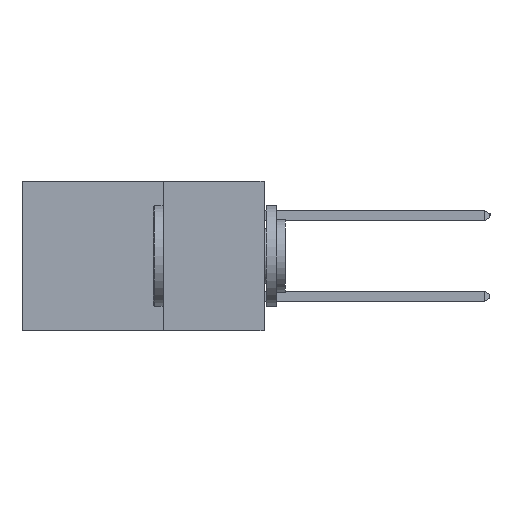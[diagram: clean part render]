
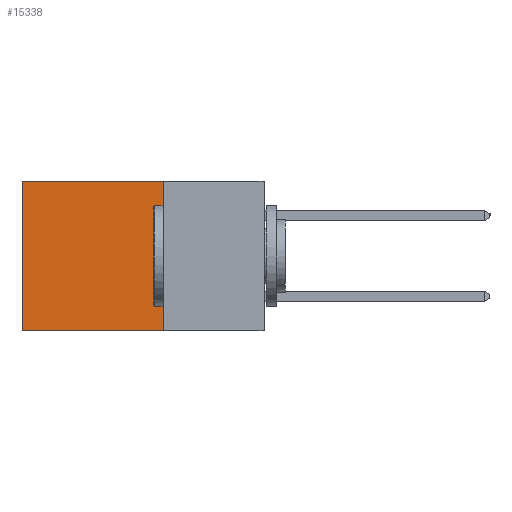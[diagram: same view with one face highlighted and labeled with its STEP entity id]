
A CAD part, left-side view. The second image highlights one B-rep face of the part: STEP entity #15338.
In plain terms, the highlighted planar face has unit normal (-1, 0, 0).
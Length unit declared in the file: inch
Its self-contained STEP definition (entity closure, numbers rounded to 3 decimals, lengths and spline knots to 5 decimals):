
#253 = LINE ( 'NONE', #8938, #17977 ) ;
#341 = VERTEX_POINT ( 'NONE', #9556 ) ;
#1748 = DIRECTION ( 'NONE',  ( 0., 0., -1. ) ) ;
#3049 = EDGE_CURVE ( 'NONE', #341, #10323, #15819, .T. ) ;
#3244 = CARTESIAN_POINT ( 'NONE',  ( 0.2615, 0.25, -0.37 ) ) ;
#3431 = DIRECTION ( 'NONE',  ( 0., 0., -1. ) ) ;
#3490 = EDGE_CURVE ( 'NONE', #7855, #14492, #253, .T. ) ;
#3608 = CARTESIAN_POINT ( 'NONE',  ( 0.2615, 0.25, -0.37 ) ) ;
#4561 = ORIENTED_EDGE ( 'NONE', *, *, #3490, .T. ) ;
#6290 = FACE_OUTER_BOUND ( 'NONE', #9276, .T. ) ;
#6962 = AXIS2_PLACEMENT_3D ( 'NONE', #10514, #20808, #3431 ) ;
#7588 = ORIENTED_EDGE ( 'NONE', *, *, #21426, .F. ) ;
#7778 = CARTESIAN_POINT ( 'NONE',  ( 0.2615, 0.6, -0.37 ) ) ;
#7855 = VERTEX_POINT ( 'NONE', #22412 ) ;
#8087 = VECTOR ( 'NONE', #1748, 39.37008 ) ;
#8106 = PLANE ( 'NONE',  #6962 ) ;
#8938 = CARTESIAN_POINT ( 'NONE',  ( 0.2615, 0.6, -0.37 ) ) ;
#9276 = EDGE_LOOP ( 'NONE', ( #4561, #7588, #12743, #11084 ) ) ;
#9556 = CARTESIAN_POINT ( 'NONE',  ( 0.2615, 0.25, 0. ) ) ;
#10323 = VERTEX_POINT ( 'NONE', #3608 ) ;
#10514 = CARTESIAN_POINT ( 'NONE',  ( 0.2615, 0.25, -0.37 ) ) ;
#11005 = CARTESIAN_POINT ( 'NONE',  ( 0.2615, 0.25, 0. ) ) ;
#11037 = VECTOR ( 'NONE', #12387, 39.37008 ) ;
#11084 = ORIENTED_EDGE ( 'NONE', *, *, #17782, .T. ) ;
#12387 = DIRECTION ( 'NONE',  ( 0., 1., 0. ) ) ;
#12743 = ORIENTED_EDGE ( 'NONE', *, *, #3049, .F. ) ;
#14492 = VERTEX_POINT ( 'NONE', #7778 ) ;
#15338 = ADVANCED_FACE ( 'NONE', ( #6290 ), #8106, .F. ) ;
#15819 = LINE ( 'NONE', #3244, #8087 ) ;
#16130 = DIRECTION ( 'NONE',  ( 0., 0., -1. ) ) ;
#16244 = DIRECTION ( 'NONE',  ( 0., 1., 0. ) ) ;
#17782 = EDGE_CURVE ( 'NONE', #341, #7855, #21314, .T. ) ;
#17977 = VECTOR ( 'NONE', #16130, 39.37008 ) ;
#19989 = LINE ( 'NONE', #21934, #20979 ) ;
#20808 = DIRECTION ( 'NONE',  ( 1., 0., 0. ) ) ;
#20979 = VECTOR ( 'NONE', #16244, 39.37008 ) ;
#21314 = LINE ( 'NONE', #11005, #11037 ) ;
#21426 = EDGE_CURVE ( 'NONE', #10323, #14492, #19989, .T. ) ;
#21934 = CARTESIAN_POINT ( 'NONE',  ( 0.2615, 0.25, -0.37 ) ) ;
#22412 = CARTESIAN_POINT ( 'NONE',  ( 0.2615, 0.6, 0. ) ) ;
